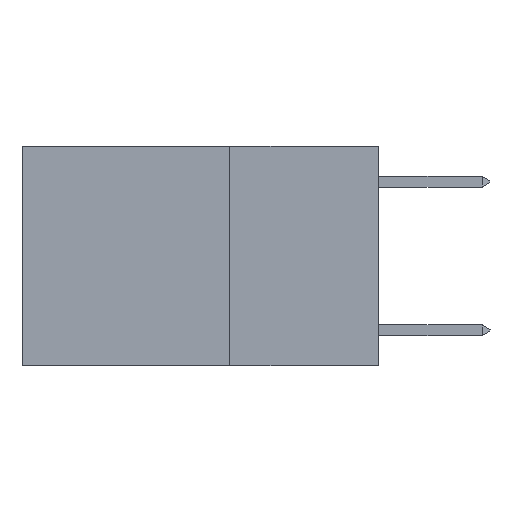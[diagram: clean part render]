
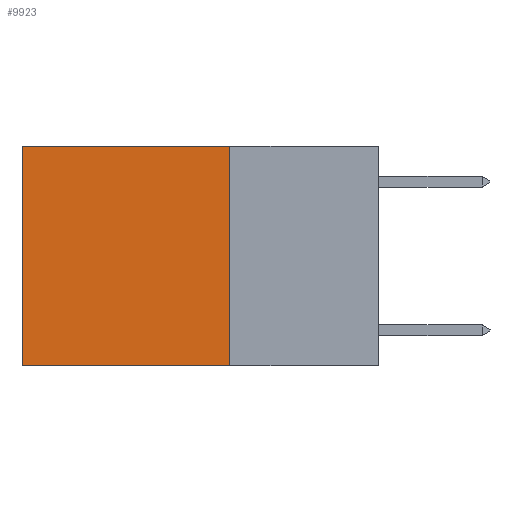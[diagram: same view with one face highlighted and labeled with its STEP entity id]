
A CAD part, left-side view. The second image highlights one B-rep face of the part: STEP entity #9923.
In plain terms, the highlighted planar face has unit normal (-1, 0, 0).
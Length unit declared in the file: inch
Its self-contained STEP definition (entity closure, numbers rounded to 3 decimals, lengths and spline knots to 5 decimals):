
#246 = EDGE_CURVE ( 'NONE', #20641, #2893, #3574, .T. ) ;
#1075 = CARTESIAN_POINT ( 'NONE',  ( 0.2625, 0.25, 0. ) ) ;
#1443 = CARTESIAN_POINT ( 'NONE',  ( 0.2625, 0.25, 0. ) ) ;
#1527 = DIRECTION ( 'NONE',  ( 1., 0., 0. ) ) ;
#2518 = CARTESIAN_POINT ( 'NONE',  ( 0.2625, 0.25, -0.37 ) ) ;
#2799 = CARTESIAN_POINT ( 'NONE',  ( 0.2625, 0.6, 0. ) ) ;
#2893 = VERTEX_POINT ( 'NONE', #4270 ) ;
#3523 = FACE_OUTER_BOUND ( 'NONE', #11879, .T. ) ;
#3574 = LINE ( 'NONE', #1443, #27777 ) ;
#3860 = DIRECTION ( 'NONE',  ( 0., 1., 0. ) ) ;
#3976 = VECTOR ( 'NONE', #17700, 39.37008 ) ;
#4270 = CARTESIAN_POINT ( 'NONE',  ( 0.2625, 0.6, 0. ) ) ;
#5115 = ORIENTED_EDGE ( 'NONE', *, *, #7821, .F. ) ;
#5922 = ORIENTED_EDGE ( 'NONE', *, *, #15075, .F. ) ;
#7759 = CARTESIAN_POINT ( 'NONE',  ( 0.2625, 0.6, -0.37 ) ) ;
#7821 = EDGE_CURVE ( 'NONE', #20641, #11837, #13322, .T. ) ;
#7936 = VERTEX_POINT ( 'NONE', #7759 ) ;
#8031 = PLANE ( 'NONE',  #14077 ) ;
#9375 = ORIENTED_EDGE ( 'NONE', *, *, #246, .T. ) ;
#9729 = LINE ( 'NONE', #2799, #13403 ) ;
#9923 = ADVANCED_FACE ( 'NONE', ( #3523 ), #8031, .F. ) ;
#11441 = DIRECTION ( 'NONE',  ( 0., 0., -1. ) ) ;
#11837 = VERTEX_POINT ( 'NONE', #13546 ) ;
#11879 = EDGE_LOOP ( 'NONE', ( #16714, #5922, #5115, #9375 ) ) ;
#13309 = LINE ( 'NONE', #2518, #3976 ) ;
#13322 = LINE ( 'NONE', #21959, #17614 ) ;
#13403 = VECTOR ( 'NONE', #11441, 39.37008 ) ;
#13546 = CARTESIAN_POINT ( 'NONE',  ( 0.2625, 0.25, -0.37 ) ) ;
#13822 = EDGE_CURVE ( 'NONE', #2893, #7936, #9729, .T. ) ;
#14077 = AXIS2_PLACEMENT_3D ( 'NONE', #20962, #1527, #27331 ) ;
#15075 = EDGE_CURVE ( 'NONE', #11837, #7936, #13309, .T. ) ;
#16714 = ORIENTED_EDGE ( 'NONE', *, *, #13822, .T. ) ;
#17614 = VECTOR ( 'NONE', #22372, 39.37008 ) ;
#17700 = DIRECTION ( 'NONE',  ( 0., 1., 0. ) ) ;
#20641 = VERTEX_POINT ( 'NONE', #1075 ) ;
#20962 = CARTESIAN_POINT ( 'NONE',  ( 0.2625, 0.25, 0. ) ) ;
#21959 = CARTESIAN_POINT ( 'NONE',  ( 0.2625, 0.25, 0. ) ) ;
#22372 = DIRECTION ( 'NONE',  ( 0., 0., -1. ) ) ;
#27331 = DIRECTION ( 'NONE',  ( 0., 0., -1. ) ) ;
#27777 = VECTOR ( 'NONE', #3860, 39.37008 ) ;
